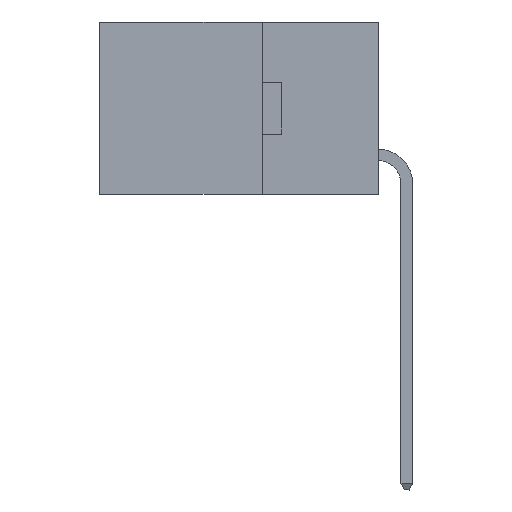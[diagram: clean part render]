
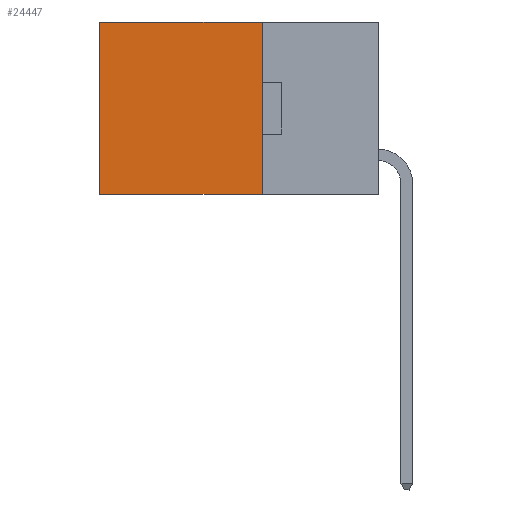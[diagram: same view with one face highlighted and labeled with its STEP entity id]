
A CAD part, left-side view. The second image highlights one B-rep face of the part: STEP entity #24447.
In plain terms, the highlighted planar face has unit normal (-1, 0, 0).
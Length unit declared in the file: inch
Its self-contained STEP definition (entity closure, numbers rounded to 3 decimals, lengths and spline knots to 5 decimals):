
#65 = CARTESIAN_POINT ( 'NONE',  ( 0.2615, 0.25, -0.37 ) ) ;
#1641 = LINE ( 'NONE', #8023, #11872 ) ;
#2042 = VERTEX_POINT ( 'NONE', #11421 ) ;
#2298 = ORIENTED_EDGE ( 'NONE', *, *, #27143, .T. ) ;
#2382 = DIRECTION ( 'NONE',  ( 1., 0., 0. ) ) ;
#4003 = DIRECTION ( 'NONE',  ( 0., 1., 0. ) ) ;
#5868 = EDGE_CURVE ( 'NONE', #16709, #9927, #10610, .T. ) ;
#8023 = CARTESIAN_POINT ( 'NONE',  ( 0.2615, 0.25, 0. ) ) ;
#8495 = EDGE_CURVE ( 'NONE', #16709, #2042, #1641, .T. ) ;
#8533 = DIRECTION ( 'NONE',  ( 0., 0., -1. ) ) ;
#8899 = DIRECTION ( 'NONE',  ( 0., 0., -1. ) ) ;
#9927 = VERTEX_POINT ( 'NONE', #17271 ) ;
#9987 = ORIENTED_EDGE ( 'NONE', *, *, #5868, .F. ) ;
#10610 = LINE ( 'NONE', #65, #19352 ) ;
#10829 = CARTESIAN_POINT ( 'NONE',  ( 0.2615, 0.25, -0.37 ) ) ;
#11421 = CARTESIAN_POINT ( 'NONE',  ( 0.2615, 0.6, 0. ) ) ;
#11872 = VECTOR ( 'NONE', #4003, 39.37008 ) ;
#12445 = EDGE_CURVE ( 'NONE', #9927, #24615, #21319, .T. ) ;
#12712 = DIRECTION ( 'NONE',  ( 0., 1., 0. ) ) ;
#13120 = CARTESIAN_POINT ( 'NONE',  ( 0.2615, 0.25, -0.37 ) ) ;
#13650 = ORIENTED_EDGE ( 'NONE', *, *, #8495, .T. ) ;
#15146 = FACE_OUTER_BOUND ( 'NONE', #15334, .T. ) ;
#15334 = EDGE_LOOP ( 'NONE', ( #2298, #16683, #9987, #13650 ) ) ;
#15445 = CARTESIAN_POINT ( 'NONE',  ( 0.2615, 0.25, 0. ) ) ;
#16392 = LINE ( 'NONE', #26945, #16878 ) ;
#16683 = ORIENTED_EDGE ( 'NONE', *, *, #12445, .F. ) ;
#16709 = VERTEX_POINT ( 'NONE', #15445 ) ;
#16878 = VECTOR ( 'NONE', #18457, 39.37008 ) ;
#17271 = CARTESIAN_POINT ( 'NONE',  ( 0.2615, 0.25, -0.37 ) ) ;
#17345 = PLANE ( 'NONE',  #20822 ) ;
#18457 = DIRECTION ( 'NONE',  ( 0., 0., -1. ) ) ;
#19352 = VECTOR ( 'NONE', #8533, 39.37008 ) ;
#20822 = AXIS2_PLACEMENT_3D ( 'NONE', #10829, #2382, #8899 ) ;
#21319 = LINE ( 'NONE', #13120, #22032 ) ;
#22032 = VECTOR ( 'NONE', #12712, 39.37008 ) ;
#22060 = CARTESIAN_POINT ( 'NONE',  ( 0.2615, 0.6, -0.37 ) ) ;
#24447 = ADVANCED_FACE ( 'NONE', ( #15146 ), #17345, .F. ) ;
#24615 = VERTEX_POINT ( 'NONE', #22060 ) ;
#26945 = CARTESIAN_POINT ( 'NONE',  ( 0.2615, 0.6, -0.37 ) ) ;
#27143 = EDGE_CURVE ( 'NONE', #2042, #24615, #16392, .T. ) ;
